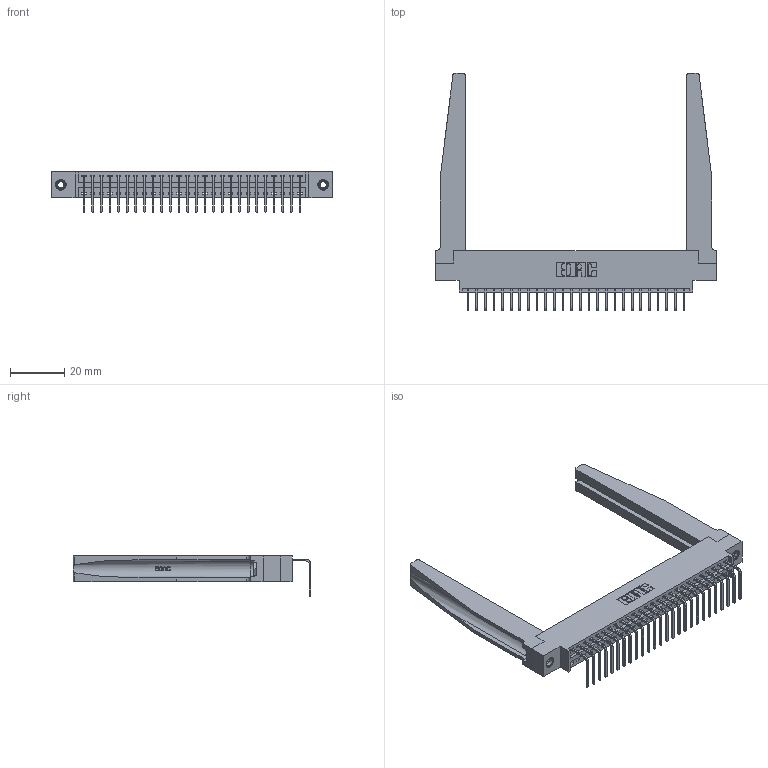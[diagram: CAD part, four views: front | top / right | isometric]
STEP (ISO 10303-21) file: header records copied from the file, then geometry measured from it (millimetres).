
FILE_DESCRIPTION (( 'STEP AP203' ), '1' );
FILE_NAME ('346-026-558-678.STEP', '2022-05-06T03:30:53', ( '' ), ( '' ), 'SwSTEP 2.0', 'SolidWorks 2020', '' );
FILE_SCHEMA (( 'CONFIG_CONTROL_DESIGN' ));
Length unit declared in the file: inch
Products named in the file (5): 346-026-558-678; 346-220-078_345-220-078; 345-250-001_345-250-001-102; 345-292-001_558 Tail - 2; 346 Part_0.170 Offset - 0.156 Dia-TH
Assembly tree (31 placements, depth 2):
  346-026-558-678
    346 Part_0.170 Offset - 0.156 Dia-TH
    345-292-001_558 Tail - 2  x26
    346-220-078_345-220-078  x2
    345-250-001_345-250-001-102  x2
Bounding box: 103.12 x 87.44 x 14.73 mm (x, y, z)
Volume: 16583.8 mm3; surface area: 19169.3 mm2
Topology: 31 solids, 31 shells, 1934 faces, 5717 edges, 3766 vertices
Faces by surface type: plane 1328, cylinder 554, bspline 36, cone 12, torus 4
Entity records: 23670 total; most frequent: CARTESIAN_POINT 4979, ORIENTED_EDGE 3826, DIRECTION 3395, EDGE_CURVE 1913, LINE 1583, VECTOR 1583, VERTEX_POINT 1268, AXIS2_PLACEMENT_3D 906
